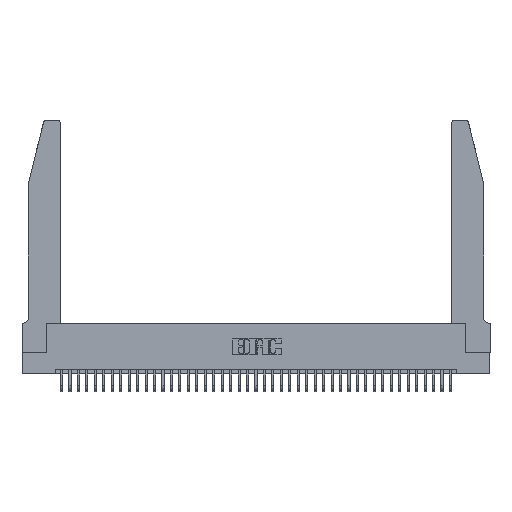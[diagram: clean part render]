
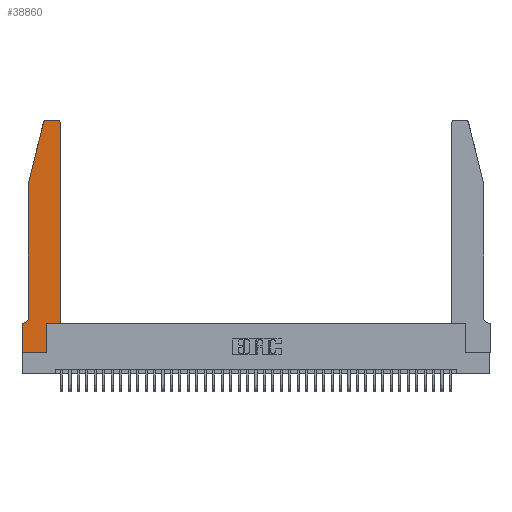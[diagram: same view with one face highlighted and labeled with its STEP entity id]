
A CAD part, top view. The second image highlights one B-rep face of the part: STEP entity #38860.
In plain terms, the highlighted planar face has unit normal (0, 0, 1).
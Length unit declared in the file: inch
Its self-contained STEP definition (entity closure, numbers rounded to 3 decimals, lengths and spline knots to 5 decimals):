
#267 = CARTESIAN_POINT ( 'NONE',  ( 0.0755, 2., 0.37 ) ) ;
#611 = CARTESIAN_POINT ( 'NONE',  ( 0.0055, 0.35, 0.37 ) ) ;
#873 = VECTOR ( 'NONE', #37091, 39.37008 ) ;
#1144 = EDGE_CURVE ( 'NONE', #20199, #31604, #18927, .T. ) ;
#1315 = CARTESIAN_POINT ( 'NONE',  ( 0., 0., 0.37 ) ) ;
#1516 = CARTESIAN_POINT ( 'NONE',  ( 0.2865, 0.35, 0.37 ) ) ;
#2105 = EDGE_CURVE ( 'NONE', #42571, #38338, #40531, .T. ) ;
#2575 = VECTOR ( 'NONE', #19673, 39.37008 ) ;
#2771 = VECTOR ( 'NONE', #7477, 39.37008 ) ;
#3224 = DIRECTION ( 'NONE',  ( -1., 0., 0. ) ) ;
#3603 = ORIENTED_EDGE ( 'NONE', *, *, #25426, .T. ) ;
#3854 = CARTESIAN_POINT ( 'NONE',  ( 0.4505, 2.72, 0.37 ) ) ;
#4232 = EDGE_CURVE ( 'NONE', #12668, #21618, #30338, .T. ) ;
#4894 = AXIS2_PLACEMENT_3D ( 'NONE', #11880, #8585, #28437 ) ;
#5551 = CARTESIAN_POINT ( 'NONE',  ( 0.0755, 2., 0.37 ) ) ;
#5667 = LINE ( 'NONE', #267, #2575 ) ;
#6364 = DIRECTION ( 'NONE',  ( 1., 0., 0. ) ) ;
#7140 = DIRECTION ( 'NONE',  ( -1., 0., 0. ) ) ;
#7302 = LINE ( 'NONE', #14017, #24790 ) ;
#7477 = DIRECTION ( 'NONE',  ( 1., 0., 0. ) ) ;
#7567 = CARTESIAN_POINT ( 'NONE',  ( 0., 0., 0.37 ) ) ;
#8018 = VECTOR ( 'NONE', #11150, 39.37008 ) ;
#8151 = ORIENTED_EDGE ( 'NONE', *, *, #41214, .T. ) ;
#8585 = DIRECTION ( 'NONE',  ( 0., 0., 1. ) ) ;
#8995 = ORIENTED_EDGE ( 'NONE', *, *, #2105, .T. ) ;
#10019 = CARTESIAN_POINT ( 'NONE',  ( 0., 0.35, 0.37 ) ) ;
#10867 = DIRECTION ( 'NONE',  ( 0., 1., 0. ) ) ;
#11150 = DIRECTION ( 'NONE',  ( 0., -1., 0. ) ) ;
#11347 = VERTEX_POINT ( 'NONE', #15272 ) ;
#11880 = CARTESIAN_POINT ( 'NONE',  ( 0.4205, 2.72, 0.37 ) ) ;
#12192 = ORIENTED_EDGE ( 'NONE', *, *, #30635, .T. ) ;
#12668 = VERTEX_POINT ( 'NONE', #32729 ) ;
#13488 = ORIENTED_EDGE ( 'NONE', *, *, #4232, .T. ) ;
#13498 = VERTEX_POINT ( 'NONE', #5551 ) ;
#13527 = CARTESIAN_POINT ( 'NONE',  ( 0.2865, 0.35, 0.37 ) ) ;
#14017 = CARTESIAN_POINT ( 'NONE',  ( 0.2605, 2.75, 0.37 ) ) ;
#14100 = EDGE_CURVE ( 'NONE', #32525, #20199, #22178, .T. ) ;
#14341 = LINE ( 'NONE', #36460, #33975 ) ;
#15272 = CARTESIAN_POINT ( 'NONE',  ( 0.4205, 2.75, 0.37 ) ) ;
#16468 = CARTESIAN_POINT ( 'NONE',  ( 0., 0., 0.37 ) ) ;
#16563 = CARTESIAN_POINT ( 'NONE',  ( 0., 0.35, 0.37 ) ) ;
#16861 = DIRECTION ( 'NONE',  ( 0., 0., -1. ) ) ;
#16954 = VERTEX_POINT ( 'NONE', #18954 ) ;
#18022 = VECTOR ( 'NONE', #3224, 39.37008 ) ;
#18186 = DIRECTION ( 'NONE',  ( 0., 0., 1. ) ) ;
#18871 = ORIENTED_EDGE ( 'NONE', *, *, #36166, .T. ) ;
#18927 = LINE ( 'NONE', #20376, #20439 ) ;
#18954 = CARTESIAN_POINT ( 'NONE',  ( 0.284, 2.75, 0.37 ) ) ;
#19468 = DIRECTION ( 'NONE',  ( 0., 0., 1. ) ) ;
#19673 = DIRECTION ( 'NONE',  ( 0., -1., 0. ) ) ;
#19976 = AXIS2_PLACEMENT_3D ( 'NONE', #16563, #19468, #6364 ) ;
#20199 = VERTEX_POINT ( 'NONE', #30546 ) ;
#20376 = CARTESIAN_POINT ( 'NONE',  ( 0.4505, 0.35, 0.37 ) ) ;
#20439 = VECTOR ( 'NONE', #10867, 39.37008 ) ;
#21127 = LINE ( 'NONE', #22924, #18022 ) ;
#21455 = LINE ( 'NONE', #13527, #873 ) ;
#21618 = VERTEX_POINT ( 'NONE', #611 ) ;
#22178 = LINE ( 'NONE', #40801, #41311 ) ;
#22405 = EDGE_CURVE ( 'NONE', #31604, #11347, #39897, .T. ) ;
#22924 = CARTESIAN_POINT ( 'NONE',  ( 0.0755, 0.35, 0.37 ) ) ;
#23579 = ORIENTED_EDGE ( 'NONE', *, *, #1144, .T. ) ;
#23786 = ORIENTED_EDGE ( 'NONE', *, *, #22405, .T. ) ;
#24790 = VECTOR ( 'NONE', #7140, 39.37008 ) ;
#25015 = AXIS2_PLACEMENT_3D ( 'NONE', #35362, #18186, #41252 ) ;
#25426 = EDGE_CURVE ( 'NONE', #13498, #12668, #5667, .T. ) ;
#26123 = ORIENTED_EDGE ( 'NONE', *, *, #14100, .T. ) ;
#26321 = EDGE_LOOP ( 'NONE', ( #28655, #12192, #40123, #3603, #13488, #18871, #8995, #8151, #40970, #26123, #23579, #23786 ) ) ;
#27311 = DIRECTION ( 'NONE',  ( -1., 0., 0. ) ) ;
#28437 = DIRECTION ( 'NONE',  ( 1., 0., 0. ) ) ;
#28655 = ORIENTED_EDGE ( 'NONE', *, *, #41778, .T. ) ;
#28737 = CARTESIAN_POINT ( 'NONE',  ( 0.25487, 2.72718, 0.37 ) ) ;
#29161 = FACE_OUTER_BOUND ( 'NONE', #26321, .T. ) ;
#29829 = VERTEX_POINT ( 'NONE', #28737 ) ;
#29915 = AXIS2_PLACEMENT_3D ( 'NONE', #40202, #16861, #27311 ) ;
#30338 = CIRCLE ( 'NONE', #29915, 0.07 ) ;
#30546 = CARTESIAN_POINT ( 'NONE',  ( 0.4505, 0.35, 0.37 ) ) ;
#30635 = EDGE_CURVE ( 'NONE', #16954, #29829, #35104, .T. ) ;
#31604 = VERTEX_POINT ( 'NONE', #3854 ) ;
#31688 = EDGE_CURVE ( 'NONE', #29829, #13498, #14341, .T. ) ;
#32525 = VERTEX_POINT ( 'NONE', #1516 ) ;
#32594 = PLANE ( 'NONE',  #19976 ) ;
#32729 = CARTESIAN_POINT ( 'NONE',  ( 0.0755, 0.42, 0.37 ) ) ;
#33975 = VECTOR ( 'NONE', #40172, 39.37008 ) ;
#34129 = CARTESIAN_POINT ( 'NONE',  ( 0.2865, 0., 0.37 ) ) ;
#34763 = DIRECTION ( 'NONE',  ( 1., 0., 0. ) ) ;
#35104 = CIRCLE ( 'NONE', #25015, 0.03 ) ;
#35362 = CARTESIAN_POINT ( 'NONE',  ( 0.284, 2.72, 0.37 ) ) ;
#36166 = EDGE_CURVE ( 'NONE', #21618, #42571, #21127, .T. ) ;
#36460 = CARTESIAN_POINT ( 'NONE',  ( 0.0755, 2., 0.37 ) ) ;
#37091 = DIRECTION ( 'NONE',  ( 0., 1., 0. ) ) ;
#38338 = VERTEX_POINT ( 'NONE', #16468 ) ;
#38860 = ADVANCED_FACE ( 'NONE', ( #29161 ), #32594, .T. ) ;
#39071 = EDGE_CURVE ( 'NONE', #39334, #32525, #21455, .T. ) ;
#39334 = VERTEX_POINT ( 'NONE', #34129 ) ;
#39897 = CIRCLE ( 'NONE', #4894, 0.03 ) ;
#40123 = ORIENTED_EDGE ( 'NONE', *, *, #31688, .T. ) ;
#40172 = DIRECTION ( 'NONE',  ( -0.239, -0.971, 0. ) ) ;
#40202 = CARTESIAN_POINT ( 'NONE',  ( 0.0055, 0.42, 0.37 ) ) ;
#40531 = LINE ( 'NONE', #7567, #8018 ) ;
#40801 = CARTESIAN_POINT ( 'NONE',  ( 0.4505, 0.35, 0.37 ) ) ;
#40970 = ORIENTED_EDGE ( 'NONE', *, *, #39071, .T. ) ;
#41214 = EDGE_CURVE ( 'NONE', #38338, #39334, #41408, .T. ) ;
#41252 = DIRECTION ( 'NONE',  ( 1., 0., 0. ) ) ;
#41311 = VECTOR ( 'NONE', #34763, 39.37008 ) ;
#41408 = LINE ( 'NONE', #1315, #2771 ) ;
#41778 = EDGE_CURVE ( 'NONE', #11347, #16954, #7302, .T. ) ;
#42571 = VERTEX_POINT ( 'NONE', #10019 ) ;
